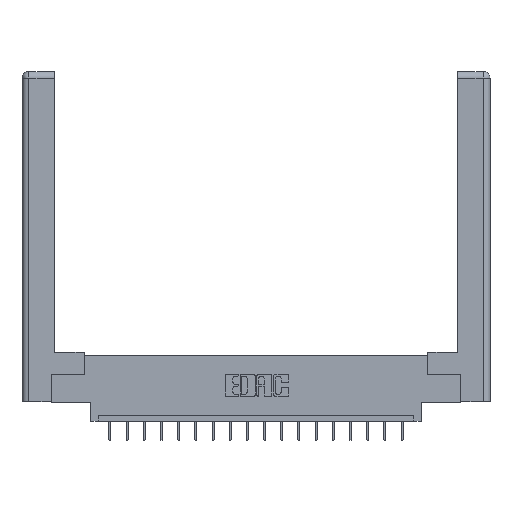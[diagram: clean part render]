
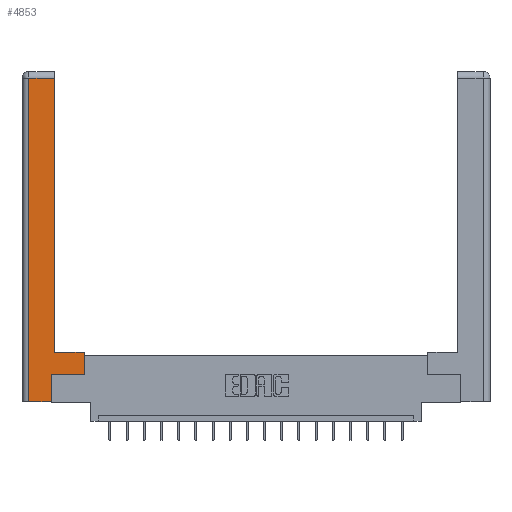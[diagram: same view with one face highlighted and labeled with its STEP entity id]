
A CAD part, top view. The second image highlights one B-rep face of the part: STEP entity #4853.
In plain terms, the highlighted planar face has unit normal (0, 0, 1).
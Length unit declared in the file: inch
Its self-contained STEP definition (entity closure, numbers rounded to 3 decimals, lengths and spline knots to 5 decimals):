
#180 = LINE ( 'NONE', #12239, #14186 ) ;
#218 = VECTOR ( 'NONE', #10836, 39.37008 ) ;
#222 = VERTEX_POINT ( 'NONE', #12954 ) ;
#264 = VERTEX_POINT ( 'NONE', #11187 ) ;
#427 = DIRECTION ( 'NONE',  ( 1., 0., 0. ) ) ;
#670 = FACE_OUTER_BOUND ( 'NONE', #8995, .T. ) ;
#780 = PLANE ( 'NONE',  #15556 ) ;
#1566 = DIRECTION ( 'NONE',  ( 0., 1., 0. ) ) ;
#1634 = VECTOR ( 'NONE', #1566, 39.37008 ) ;
#2010 = CARTESIAN_POINT ( 'NONE',  ( 0.265, 0., 0. ) ) ;
#2782 = VERTEX_POINT ( 'NONE', #14913 ) ;
#2916 = LINE ( 'NONE', #12397, #12019 ) ;
#2918 = VECTOR ( 'NONE', #9739, 39.37008 ) ;
#3055 = EDGE_CURVE ( 'NONE', #18559, #2782, #18462, .T. ) ;
#3086 = EDGE_CURVE ( 'NONE', #264, #11912, #10586, .T. ) ;
#3613 = DIRECTION ( 'NONE',  ( -1., 0., 0. ) ) ;
#3769 = LINE ( 'NONE', #4986, #4942 ) ;
#4850 = CARTESIAN_POINT ( 'NONE',  ( 0.295, 2.94, 0. ) ) ;
#4853 = ADVANCED_FACE ( 'NONE', ( #670 ), #780, .F. ) ;
#4942 = VECTOR ( 'NONE', #15413, 39.37008 ) ;
#4986 = CARTESIAN_POINT ( 'NONE',  ( 0.265, 0.245, 0. ) ) ;
#5050 = CARTESIAN_POINT ( 'NONE',  ( 0., 0., 0. ) ) ;
#6103 = CARTESIAN_POINT ( 'NONE',  ( 0.565, 0.45, 0. ) ) ;
#6471 = CARTESIAN_POINT ( 'NONE',  ( 0.265, 0.245, 0. ) ) ;
#6907 = EDGE_CURVE ( 'NONE', #9606, #12026, #11561, .T. ) ;
#6980 = CARTESIAN_POINT ( 'NONE',  ( 0.265, 0., 0. ) ) ;
#7335 = VERTEX_POINT ( 'NONE', #6471 ) ;
#7497 = VECTOR ( 'NONE', #18168, 39.37008 ) ;
#8402 = ORIENTED_EDGE ( 'NONE', *, *, #9729, .T. ) ;
#8995 = EDGE_LOOP ( 'NONE', ( #8402, #15152, #13549, #19313, #16216, #15434, #11047, #10402 ) ) ;
#9324 = DIRECTION ( 'NONE',  ( 0., 1., 0. ) ) ;
#9606 = VERTEX_POINT ( 'NONE', #15125 ) ;
#9729 = EDGE_CURVE ( 'NONE', #222, #18559, #10520, .T. ) ;
#9739 = DIRECTION ( 'NONE',  ( 1., 0., 0. ) ) ;
#9941 = EDGE_CURVE ( 'NONE', #11912, #222, #13291, .T. ) ;
#10402 = ORIENTED_EDGE ( 'NONE', *, *, #9941, .T. ) ;
#10520 = LINE ( 'NONE', #13493, #1634 ) ;
#10586 = LINE ( 'NONE', #16658, #14499 ) ;
#10836 = DIRECTION ( 'NONE',  ( -1., 0., 0. ) ) ;
#11047 = ORIENTED_EDGE ( 'NONE', *, *, #3086, .T. ) ;
#11132 = DIRECTION ( 'NONE',  ( 0., 0., -1. ) ) ;
#11187 = CARTESIAN_POINT ( 'NONE',  ( 0.565, 0.245, 0. ) ) ;
#11561 = LINE ( 'NONE', #6980, #2918 ) ;
#11912 = VERTEX_POINT ( 'NONE', #6103 ) ;
#12019 = VECTOR ( 'NONE', #16945, 39.37008 ) ;
#12026 = VERTEX_POINT ( 'NONE', #2010 ) ;
#12239 = CARTESIAN_POINT ( 'NONE',  ( 0.565, 0.245, 0. ) ) ;
#12397 = CARTESIAN_POINT ( 'NONE',  ( 0.0615, 0., 0. ) ) ;
#12954 = CARTESIAN_POINT ( 'NONE',  ( 0.295, 0.45, 0. ) ) ;
#13291 = LINE ( 'NONE', #13557, #218 ) ;
#13493 = CARTESIAN_POINT ( 'NONE',  ( 0.295, 3., 0. ) ) ;
#13512 = EDGE_CURVE ( 'NONE', #12026, #7335, #3769, .T. ) ;
#13549 = ORIENTED_EDGE ( 'NONE', *, *, #19250, .T. ) ;
#13557 = CARTESIAN_POINT ( 'NONE',  ( 0.295, 0.45, 0. ) ) ;
#14186 = VECTOR ( 'NONE', #427, 39.37008 ) ;
#14499 = VECTOR ( 'NONE', #9324, 39.37008 ) ;
#14913 = CARTESIAN_POINT ( 'NONE',  ( 0.0615, 2.94, 0. ) ) ;
#15125 = CARTESIAN_POINT ( 'NONE',  ( 0.0615, 0., 0. ) ) ;
#15152 = ORIENTED_EDGE ( 'NONE', *, *, #3055, .T. ) ;
#15413 = DIRECTION ( 'NONE',  ( 0., 1., 0. ) ) ;
#15434 = ORIENTED_EDGE ( 'NONE', *, *, #17696, .T. ) ;
#15556 = AXIS2_PLACEMENT_3D ( 'NONE', #5050, #11132, #3613 ) ;
#16216 = ORIENTED_EDGE ( 'NONE', *, *, #13512, .T. ) ;
#16597 = CARTESIAN_POINT ( 'NONE',  ( 0.0615, 2.94, 0. ) ) ;
#16658 = CARTESIAN_POINT ( 'NONE',  ( 0.565, 0.45, 0. ) ) ;
#16945 = DIRECTION ( 'NONE',  ( 0., -1., 0. ) ) ;
#17696 = EDGE_CURVE ( 'NONE', #7335, #264, #180, .T. ) ;
#18168 = DIRECTION ( 'NONE',  ( -1., 0., 0. ) ) ;
#18462 = LINE ( 'NONE', #16597, #7497 ) ;
#18559 = VERTEX_POINT ( 'NONE', #4850 ) ;
#19250 = EDGE_CURVE ( 'NONE', #2782, #9606, #2916, .T. ) ;
#19313 = ORIENTED_EDGE ( 'NONE', *, *, #6907, .T. ) ;
